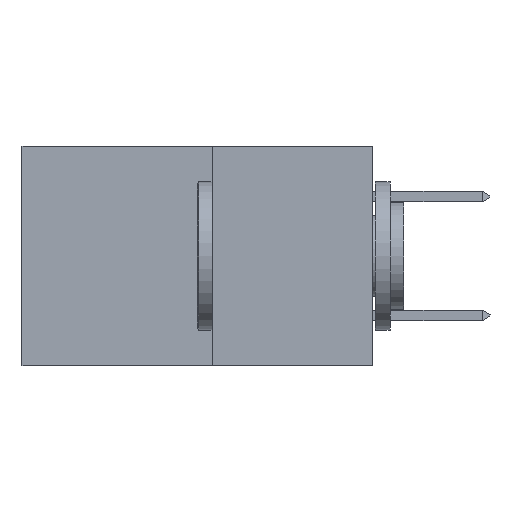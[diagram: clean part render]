
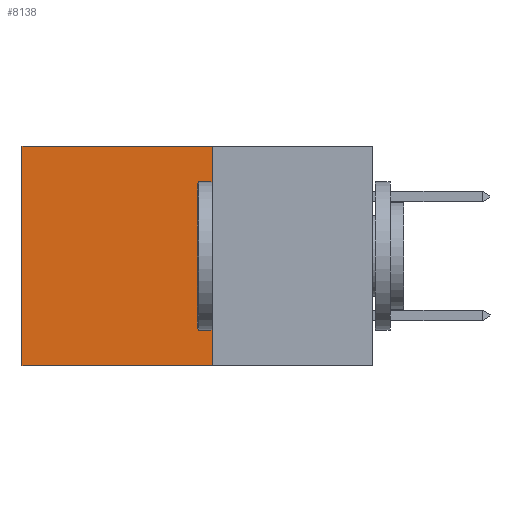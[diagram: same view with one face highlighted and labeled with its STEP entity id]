
A CAD part, left-side view. The second image highlights one B-rep face of the part: STEP entity #8138.
In plain terms, the highlighted planar face has unit normal (-1, 0, 0).
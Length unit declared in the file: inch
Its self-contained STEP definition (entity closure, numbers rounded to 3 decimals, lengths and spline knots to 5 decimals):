
#801 = CARTESIAN_POINT ( 'NONE',  ( 0.277, 0.59, -0.37 ) ) ;
#1478 = EDGE_CURVE ( 'NONE', #6565, #24671, #3864, .T. ) ;
#1555 = EDGE_CURVE ( 'NONE', #24671, #16224, #12630, .T. ) ;
#1594 = ORIENTED_EDGE ( 'NONE', *, *, #11524, .T. ) ;
#2834 = EDGE_CURVE ( 'NONE', #6565, #12180, #21924, .T. ) ;
#2918 = DIRECTION ( 'NONE',  ( 0., 0., -1. ) ) ;
#3087 = CARTESIAN_POINT ( 'NONE',  ( 0.277, 0.27, -0.37 ) ) ;
#3625 = DIRECTION ( 'NONE',  ( 1., 0., 0. ) ) ;
#3864 = LINE ( 'NONE', #13610, #24956 ) ;
#6020 = VECTOR ( 'NONE', #8450, 39.37008 ) ;
#6565 = VERTEX_POINT ( 'NONE', #25089 ) ;
#6589 = CARTESIAN_POINT ( 'NONE',  ( 0.277, 0.27, -0.37 ) ) ;
#7410 = EDGE_LOOP ( 'NONE', ( #1594, #11321, #16686, #25141 ) ) ;
#8138 = ADVANCED_FACE ( 'NONE', ( #10991 ), #11585, .F. ) ;
#8450 = DIRECTION ( 'NONE',  ( 0., 1., 0. ) ) ;
#10991 = FACE_OUTER_BOUND ( 'NONE', #7410, .T. ) ;
#11321 = ORIENTED_EDGE ( 'NONE', *, *, #1555, .F. ) ;
#11524 = EDGE_CURVE ( 'NONE', #12180, #16224, #22667, .T. ) ;
#11585 = PLANE ( 'NONE',  #24433 ) ;
#12180 = VERTEX_POINT ( 'NONE', #17422 ) ;
#12630 = LINE ( 'NONE', #6589, #22539 ) ;
#13610 = CARTESIAN_POINT ( 'NONE',  ( 0.277, 0.27, -0.37 ) ) ;
#14730 = CARTESIAN_POINT ( 'NONE',  ( 0.277, 0.59, -0.37 ) ) ;
#15588 = CARTESIAN_POINT ( 'NONE',  ( 0.277, 0.27, -0.37 ) ) ;
#16224 = VERTEX_POINT ( 'NONE', #14730 ) ;
#16686 = ORIENTED_EDGE ( 'NONE', *, *, #1478, .F. ) ;
#16767 = DIRECTION ( 'NONE',  ( 0., 0., -1. ) ) ;
#16811 = VECTOR ( 'NONE', #16767, 39.37008 ) ;
#17422 = CARTESIAN_POINT ( 'NONE',  ( 0.277, 0.59, 0. ) ) ;
#17606 = DIRECTION ( 'NONE',  ( 0., 0., -1. ) ) ;
#21924 = LINE ( 'NONE', #22732, #6020 ) ;
#22539 = VECTOR ( 'NONE', #23452, 39.37008 ) ;
#22667 = LINE ( 'NONE', #801, #16811 ) ;
#22732 = CARTESIAN_POINT ( 'NONE',  ( 0.277, 0.27, 0. ) ) ;
#23452 = DIRECTION ( 'NONE',  ( 0., 1., 0. ) ) ;
#24433 = AXIS2_PLACEMENT_3D ( 'NONE', #15588, #3625, #17606 ) ;
#24671 = VERTEX_POINT ( 'NONE', #3087 ) ;
#24956 = VECTOR ( 'NONE', #2918, 39.37008 ) ;
#25089 = CARTESIAN_POINT ( 'NONE',  ( 0.277, 0.27, 0. ) ) ;
#25141 = ORIENTED_EDGE ( 'NONE', *, *, #2834, .T. ) ;
